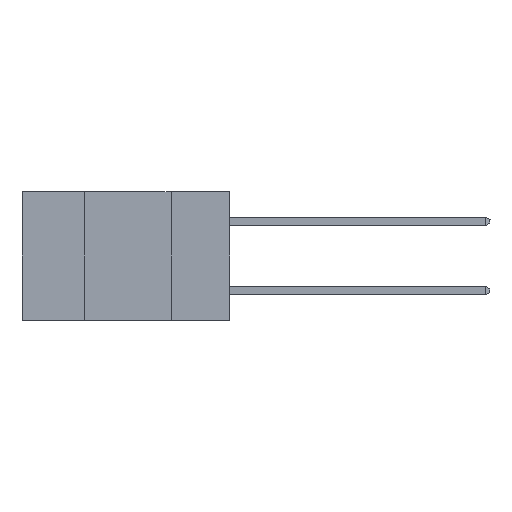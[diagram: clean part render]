
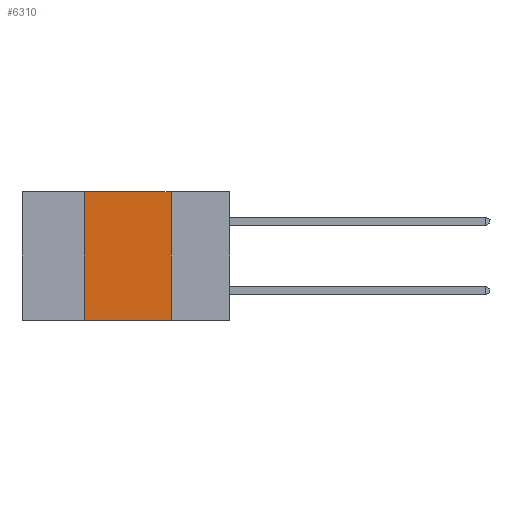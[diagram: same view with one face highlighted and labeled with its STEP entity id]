
A CAD part, left-side view. The second image highlights one B-rep face of the part: STEP entity #6310.
In plain terms, the highlighted planar face has unit normal (-1, 0, 0).
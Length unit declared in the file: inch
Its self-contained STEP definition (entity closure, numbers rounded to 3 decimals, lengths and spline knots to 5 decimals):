
#99 = EDGE_CURVE ( 'NONE', #6064, #29500, #5660, .T. ) ;
#390 = ORIENTED_EDGE ( 'NONE', *, *, #29808, .F. ) ;
#1424 = CARTESIAN_POINT ( 'NONE',  ( 0., 0.42, 0. ) ) ;
#1939 = CARTESIAN_POINT ( 'NONE',  ( 0., 0.6, 0. ) ) ;
#2879 = CARTESIAN_POINT ( 'NONE',  ( 0., 0.6, -0.37 ) ) ;
#3076 = VECTOR ( 'NONE', #5107, 39.37008 ) ;
#3095 = DIRECTION ( 'NONE',  ( 0., -1., 0. ) ) ;
#3565 = VECTOR ( 'NONE', #10749, 39.37008 ) ;
#4488 = EDGE_CURVE ( 'NONE', #20465, #12607, #18310, .T. ) ;
#4681 = EDGE_CURVE ( 'NONE', #12607, #29500, #9387, .T. ) ;
#5107 = DIRECTION ( 'NONE',  ( 0., 0., -1. ) ) ;
#5660 = LINE ( 'NONE', #2879, #23874 ) ;
#6064 = VERTEX_POINT ( 'NONE', #29842 ) ;
#6310 = ADVANCED_FACE ( 'NONE', ( #9300 ), #25535, .F. ) ;
#9300 = FACE_OUTER_BOUND ( 'NONE', #26064, .T. ) ;
#9387 = LINE ( 'NONE', #25189, #3076 ) ;
#10749 = DIRECTION ( 'NONE',  ( 0., 0., 1. ) ) ;
#11342 = DIRECTION ( 'NONE',  ( 1., 0., 0. ) ) ;
#11408 = CARTESIAN_POINT ( 'NONE',  ( 0., 0.42, 0. ) ) ;
#12607 = VERTEX_POINT ( 'NONE', #16058 ) ;
#13352 = AXIS2_PLACEMENT_3D ( 'NONE', #30348, #11342, #13712 ) ;
#13712 = DIRECTION ( 'NONE',  ( 0., 0., -1. ) ) ;
#14205 = VECTOR ( 'NONE', #16454, 39.37008 ) ;
#15665 = CARTESIAN_POINT ( 'NONE',  ( 0., 0.17, -0.37 ) ) ;
#16058 = CARTESIAN_POINT ( 'NONE',  ( 0., 0.17, 0. ) ) ;
#16454 = DIRECTION ( 'NONE',  ( 0., -1., 0. ) ) ;
#18310 = LINE ( 'NONE', #1939, #14205 ) ;
#18902 = ORIENTED_EDGE ( 'NONE', *, *, #99, .T. ) ;
#20267 = ORIENTED_EDGE ( 'NONE', *, *, #4488, .F. ) ;
#20465 = VERTEX_POINT ( 'NONE', #11408 ) ;
#20613 = LINE ( 'NONE', #1424, #3565 ) ;
#23874 = VECTOR ( 'NONE', #3095, 39.37008 ) ;
#25189 = CARTESIAN_POINT ( 'NONE',  ( 0., 0.17, 0. ) ) ;
#25535 = PLANE ( 'NONE',  #13352 ) ;
#26064 = EDGE_LOOP ( 'NONE', ( #29048, #20267, #390, #18902 ) ) ;
#29048 = ORIENTED_EDGE ( 'NONE', *, *, #4681, .F. ) ;
#29500 = VERTEX_POINT ( 'NONE', #15665 ) ;
#29808 = EDGE_CURVE ( 'NONE', #6064, #20465, #20613, .T. ) ;
#29842 = CARTESIAN_POINT ( 'NONE',  ( 0., 0.42, -0.37 ) ) ;
#30348 = CARTESIAN_POINT ( 'NONE',  ( 0., 0.6, 0. ) ) ;
